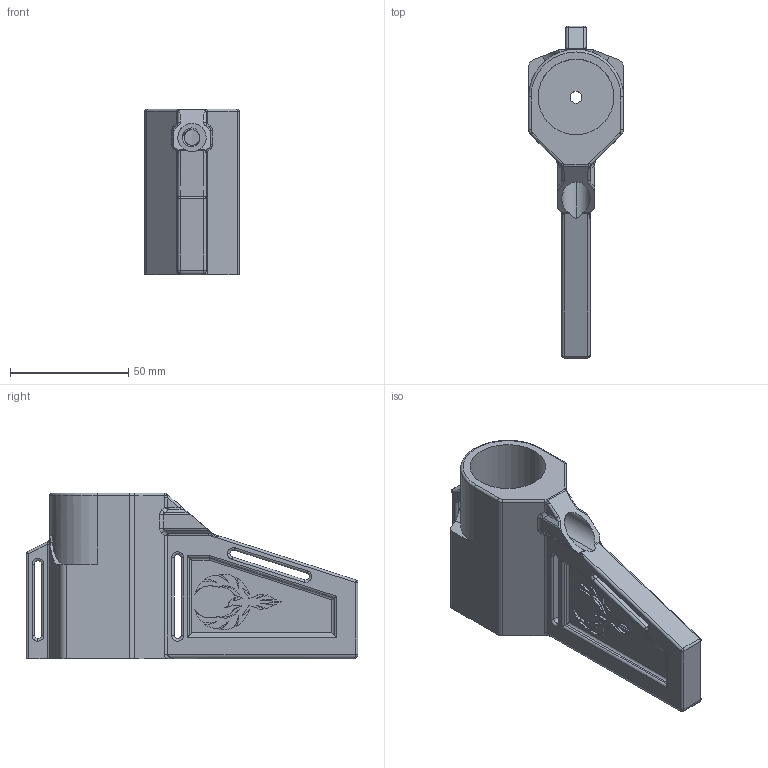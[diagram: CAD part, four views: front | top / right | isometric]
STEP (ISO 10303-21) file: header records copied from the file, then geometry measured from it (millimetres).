
FILE_DESCRIPTION (( 'STEP AP214' ), '1' );
FILE_NAME ('Spectre Mini Shockwave Brace.STEP', '2020-08-26T02:18:15', ( '' ), ( '' ), 'SwSTEP 2.0', 'SolidWorks 2019', '' );
FILE_SCHEMA (( 'AUTOMOTIVE_DESIGN' ));
Length unit declared in the file: millimetre
Products named in the file (1): Spectre Mini Shockwave Brace
Bounding box: 40 x 140.12 x 70 mm (x, y, z)
Volume: 97730.9 mm3; surface area: 34362 mm2
Topology: 1 solids, 1 shells, 1550 faces, 4529 edges, 2976 vertices
Faces by surface type: plane 1350, cylinder 122, bspline 55, torus 19, sphere 4
Entity records: 56630 total; most frequent: CARTESIAN_POINT 15960, ORIENTED_EDGE 9038, DIRECTION 7467, EDGE_CURVE 4519, VECTOR 4159, LINE 4159, VERTEX_POINT 2976, AXIS2_PLACEMENT_3D 1654
